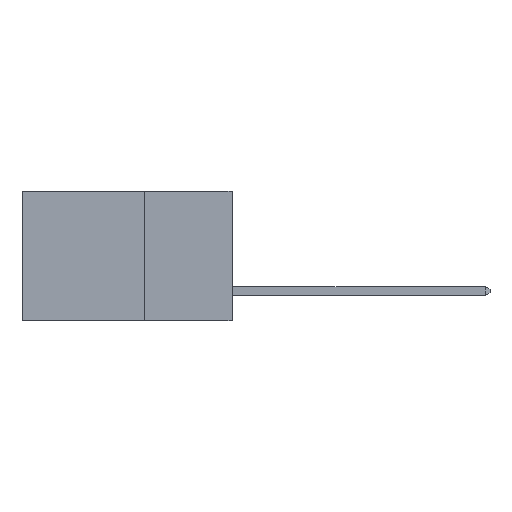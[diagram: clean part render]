
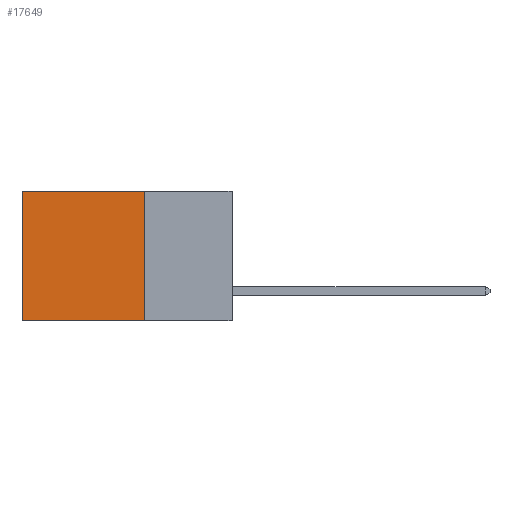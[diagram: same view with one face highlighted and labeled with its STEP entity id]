
A CAD part, left-side view. The second image highlights one B-rep face of the part: STEP entity #17649.
In plain terms, the highlighted planar face has unit normal (-1, 0, 0).
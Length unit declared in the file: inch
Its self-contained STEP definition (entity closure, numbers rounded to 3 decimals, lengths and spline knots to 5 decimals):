
#581 = CARTESIAN_POINT ( 'NONE',  ( 0.2875, 0.25, 0. ) ) ;
#661 = ORIENTED_EDGE ( 'NONE', *, *, #10245, .T. ) ;
#706 = CARTESIAN_POINT ( 'NONE',  ( 0.2875, 0.25, 0. ) ) ;
#839 = DIRECTION ( 'NONE',  ( 0., 0., -1. ) ) ;
#1207 = DIRECTION ( 'NONE',  ( 0., 1., 0. ) ) ;
#1360 = VERTEX_POINT ( 'NONE', #12956 ) ;
#3311 = VECTOR ( 'NONE', #6046, 39.37008 ) ;
#3606 = VECTOR ( 'NONE', #839, 39.37008 ) ;
#4285 = CARTESIAN_POINT ( 'NONE',  ( 0.2875, 0.25, -0.37 ) ) ;
#5406 = DIRECTION ( 'NONE',  ( 0., 0., -1. ) ) ;
#5639 = EDGE_CURVE ( 'NONE', #5923, #1360, #10946, .T. ) ;
#5923 = VERTEX_POINT ( 'NONE', #581 ) ;
#6025 = VERTEX_POINT ( 'NONE', #6956 ) ;
#6046 = DIRECTION ( 'NONE',  ( 0., 1., 0. ) ) ;
#6956 = CARTESIAN_POINT ( 'NONE',  ( 0.2875, 0.6, -0.37 ) ) ;
#7595 = EDGE_LOOP ( 'NONE', ( #661, #13487, #12513, #10528 ) ) ;
#7672 = LINE ( 'NONE', #17526, #3606 ) ;
#8397 = PLANE ( 'NONE',  #17941 ) ;
#8736 = DIRECTION ( 'NONE',  ( 0., 0., -1. ) ) ;
#10245 = EDGE_CURVE ( 'NONE', #1360, #6025, #7672, .T. ) ;
#10283 = VERTEX_POINT ( 'NONE', #11661 ) ;
#10322 = EDGE_CURVE ( 'NONE', #5923, #10283, #10788, .T. ) ;
#10528 = ORIENTED_EDGE ( 'NONE', *, *, #5639, .T. ) ;
#10788 = LINE ( 'NONE', #16218, #14782 ) ;
#10946 = LINE ( 'NONE', #16566, #3311 ) ;
#11661 = CARTESIAN_POINT ( 'NONE',  ( 0.2875, 0.25, -0.37 ) ) ;
#11846 = FACE_OUTER_BOUND ( 'NONE', #7595, .T. ) ;
#12513 = ORIENTED_EDGE ( 'NONE', *, *, #10322, .F. ) ;
#12956 = CARTESIAN_POINT ( 'NONE',  ( 0.2875, 0.6, 0. ) ) ;
#13487 = ORIENTED_EDGE ( 'NONE', *, *, #13865, .F. ) ;
#13865 = EDGE_CURVE ( 'NONE', #10283, #6025, #18731, .T. ) ;
#14473 = DIRECTION ( 'NONE',  ( 1., 0., 0. ) ) ;
#14782 = VECTOR ( 'NONE', #8736, 39.37008 ) ;
#16218 = CARTESIAN_POINT ( 'NONE',  ( 0.2875, 0.25, 0. ) ) ;
#16566 = CARTESIAN_POINT ( 'NONE',  ( 0.2875, 0.25, 0. ) ) ;
#17526 = CARTESIAN_POINT ( 'NONE',  ( 0.2875, 0.6, 0. ) ) ;
#17649 = ADVANCED_FACE ( 'NONE', ( #11846 ), #8397, .F. ) ;
#17941 = AXIS2_PLACEMENT_3D ( 'NONE', #706, #14473, #5406 ) ;
#18275 = VECTOR ( 'NONE', #1207, 39.37008 ) ;
#18731 = LINE ( 'NONE', #4285, #18275 ) ;
